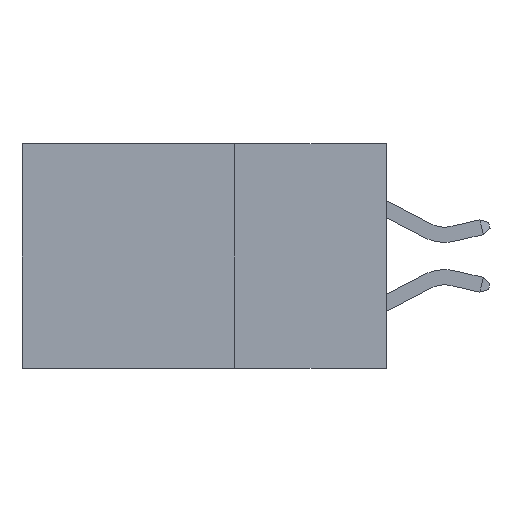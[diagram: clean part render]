
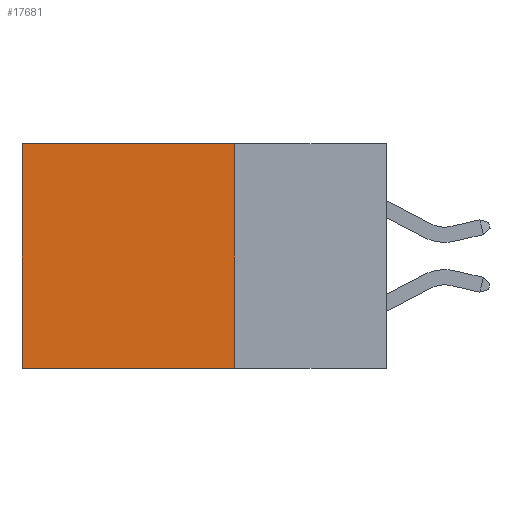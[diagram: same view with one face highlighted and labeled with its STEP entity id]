
A CAD part, left-side view. The second image highlights one B-rep face of the part: STEP entity #17681.
In plain terms, the highlighted planar face has unit normal (-1, 0, 0).
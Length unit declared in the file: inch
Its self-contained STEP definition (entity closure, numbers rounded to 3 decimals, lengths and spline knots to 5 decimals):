
#4 = LINE ( 'NONE', #3105, #17958 ) ;
#374 = ORIENTED_EDGE ( 'NONE', *, *, #18174, .T. ) ;
#476 = VECTOR ( 'NONE', #12534, 39.37008 ) ;
#605 = CARTESIAN_POINT ( 'NONE',  ( 0.2615, 0.6, 0. ) ) ;
#1086 = CARTESIAN_POINT ( 'NONE',  ( 0.2615, 0.25, 0. ) ) ;
#1304 = LINE ( 'NONE', #5800, #13105 ) ;
#1525 = AXIS2_PLACEMENT_3D ( 'NONE', #17473, #10622, #17156 ) ;
#2054 = EDGE_CURVE ( 'NONE', #4830, #11113, #1304, .T. ) ;
#3105 = CARTESIAN_POINT ( 'NONE',  ( 0.2615, 0.25, -0.37 ) ) ;
#4830 = VERTEX_POINT ( 'NONE', #16078 ) ;
#5800 = CARTESIAN_POINT ( 'NONE',  ( 0.2615, 0.25, -0.37 ) ) ;
#5878 = CARTESIAN_POINT ( 'NONE',  ( 0.2615, 0.6, -0.37 ) ) ;
#8876 = DIRECTION ( 'NONE',  ( 0., 0., -1. ) ) ;
#9814 = VERTEX_POINT ( 'NONE', #605 ) ;
#10622 = DIRECTION ( 'NONE',  ( 1., 0., 0. ) ) ;
#11113 = VERTEX_POINT ( 'NONE', #12149 ) ;
#11971 = VERTEX_POINT ( 'NONE', #18246 ) ;
#12149 = CARTESIAN_POINT ( 'NONE',  ( 0.2615, 0.6, -0.37 ) ) ;
#12412 = ORIENTED_EDGE ( 'NONE', *, *, #18590, .T. ) ;
#12534 = DIRECTION ( 'NONE',  ( 0., 1., 0. ) ) ;
#13105 = VECTOR ( 'NONE', #20434, 39.37008 ) ;
#14160 = FACE_OUTER_BOUND ( 'NONE', #16232, .T. ) ;
#14552 = EDGE_CURVE ( 'NONE', #11971, #4830, #4, .T. ) ;
#15604 = ORIENTED_EDGE ( 'NONE', *, *, #14552, .F. ) ;
#15715 = LINE ( 'NONE', #5878, #20625 ) ;
#15826 = DIRECTION ( 'NONE',  ( 0., 0., -1. ) ) ;
#16078 = CARTESIAN_POINT ( 'NONE',  ( 0.2615, 0.25, -0.37 ) ) ;
#16232 = EDGE_LOOP ( 'NONE', ( #12412, #18785, #15604, #374 ) ) ;
#17156 = DIRECTION ( 'NONE',  ( 0., 0., -1. ) ) ;
#17237 = LINE ( 'NONE', #1086, #476 ) ;
#17473 = CARTESIAN_POINT ( 'NONE',  ( 0.2615, 0.25, -0.37 ) ) ;
#17573 = PLANE ( 'NONE',  #1525 ) ;
#17681 = ADVANCED_FACE ( 'NONE', ( #14160 ), #17573, .F. ) ;
#17958 = VECTOR ( 'NONE', #15826, 39.37008 ) ;
#18174 = EDGE_CURVE ( 'NONE', #11971, #9814, #17237, .T. ) ;
#18246 = CARTESIAN_POINT ( 'NONE',  ( 0.2615, 0.25, 0. ) ) ;
#18590 = EDGE_CURVE ( 'NONE', #9814, #11113, #15715, .T. ) ;
#18785 = ORIENTED_EDGE ( 'NONE', *, *, #2054, .F. ) ;
#20434 = DIRECTION ( 'NONE',  ( 0., 1., 0. ) ) ;
#20625 = VECTOR ( 'NONE', #8876, 39.37008 ) ;
